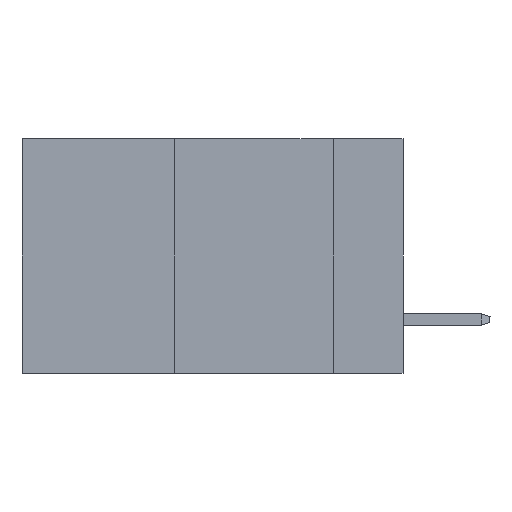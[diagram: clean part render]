
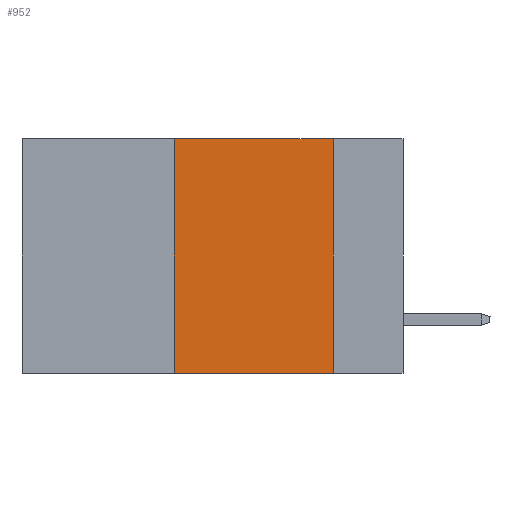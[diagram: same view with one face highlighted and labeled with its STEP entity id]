
A CAD part, left-side view. The second image highlights one B-rep face of the part: STEP entity #952.
In plain terms, the highlighted planar face has unit normal (-1, 0, 0).
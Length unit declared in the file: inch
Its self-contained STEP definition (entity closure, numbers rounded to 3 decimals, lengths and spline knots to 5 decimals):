
#952 = ADVANCED_FACE ( 'NONE', ( #19545 ), #16441, .F. ) ;
#1504 = DIRECTION ( 'NONE',  ( 1., 0., 0. ) ) ;
#2368 = ORIENTED_EDGE ( 'NONE', *, *, #12317, .F. ) ;
#2646 = DIRECTION ( 'NONE',  ( 0., -1., 0. ) ) ;
#2953 = ORIENTED_EDGE ( 'NONE', *, *, #19046, .T. ) ;
#3167 = DIRECTION ( 'NONE',  ( 0., 0., 1. ) ) ;
#3262 = DIRECTION ( 'NONE',  ( 0., 0., -1. ) ) ;
#3801 = CARTESIAN_POINT ( 'NONE',  ( 0., 0.36, 0. ) ) ;
#3868 = CARTESIAN_POINT ( 'NONE',  ( 0., 0.36, -0.37 ) ) ;
#4387 = LINE ( 'NONE', #9153, #16720 ) ;
#5923 = LINE ( 'NONE', #10860, #11213 ) ;
#8432 = CARTESIAN_POINT ( 'NONE',  ( 0., 0.11, -0.37 ) ) ;
#9153 = CARTESIAN_POINT ( 'NONE',  ( 0., 0.6, -0.37 ) ) ;
#9383 = DIRECTION ( 'NONE',  ( 0., 0., -1. ) ) ;
#10860 = CARTESIAN_POINT ( 'NONE',  ( 0., 0.6, 0. ) ) ;
#11015 = EDGE_CURVE ( 'NONE', #30113, #18322, #15895, .T. ) ;
#11213 = VECTOR ( 'NONE', #2646, 39.37008 ) ;
#12317 = EDGE_CURVE ( 'NONE', #22675, #30113, #5923, .T. ) ;
#12396 = VECTOR ( 'NONE', #3167, 39.37008 ) ;
#12886 = VERTEX_POINT ( 'NONE', #3868 ) ;
#13504 = CARTESIAN_POINT ( 'NONE',  ( 0., 0.36, 0. ) ) ;
#14630 = CARTESIAN_POINT ( 'NONE',  ( 0., 0.6, 0. ) ) ;
#15895 = LINE ( 'NONE', #28497, #30578 ) ;
#16441 = PLANE ( 'NONE',  #25513 ) ;
#16720 = VECTOR ( 'NONE', #21482, 39.37008 ) ;
#17421 = ORIENTED_EDGE ( 'NONE', *, *, #11015, .F. ) ;
#18322 = VERTEX_POINT ( 'NONE', #8432 ) ;
#19046 = EDGE_CURVE ( 'NONE', #12886, #18322, #4387, .T. ) ;
#19545 = FACE_OUTER_BOUND ( 'NONE', #22842, .T. ) ;
#20554 = LINE ( 'NONE', #13504, #12396 ) ;
#21482 = DIRECTION ( 'NONE',  ( 0., -1., 0. ) ) ;
#22675 = VERTEX_POINT ( 'NONE', #3801 ) ;
#22842 = EDGE_LOOP ( 'NONE', ( #17421, #2368, #26047, #2953 ) ) ;
#25513 = AXIS2_PLACEMENT_3D ( 'NONE', #14630, #1504, #9383 ) ;
#26047 = ORIENTED_EDGE ( 'NONE', *, *, #30833, .F. ) ;
#28272 = CARTESIAN_POINT ( 'NONE',  ( 0., 0.11, 0. ) ) ;
#28497 = CARTESIAN_POINT ( 'NONE',  ( 0., 0.11, 0. ) ) ;
#30113 = VERTEX_POINT ( 'NONE', #28272 ) ;
#30578 = VECTOR ( 'NONE', #3262, 39.37008 ) ;
#30833 = EDGE_CURVE ( 'NONE', #12886, #22675, #20554, .T. ) ;
